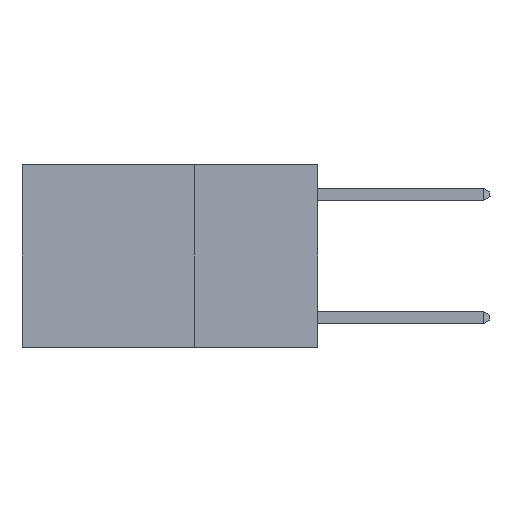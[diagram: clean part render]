
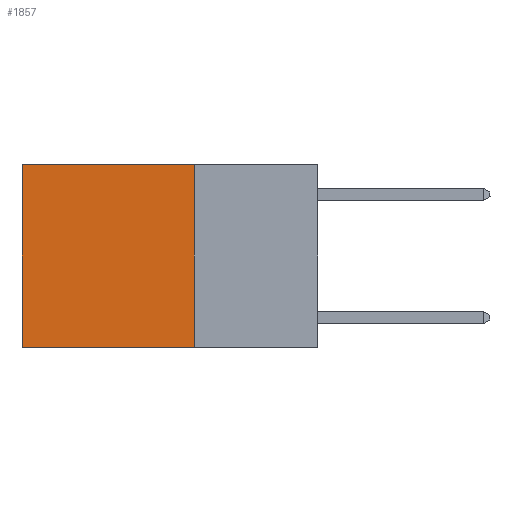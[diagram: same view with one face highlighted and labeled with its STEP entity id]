
A CAD part, left-side view. The second image highlights one B-rep face of the part: STEP entity #1857.
In plain terms, the highlighted planar face has unit normal (-1, 0, 0).
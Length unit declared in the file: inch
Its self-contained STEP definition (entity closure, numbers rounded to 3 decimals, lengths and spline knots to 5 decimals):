
#197 = CARTESIAN_POINT ( 'NONE',  ( 0.2625, 0.25, -0.37 ) ) ;
#1006 = LINE ( 'NONE', #4265, #3713 ) ;
#1363 = CARTESIAN_POINT ( 'NONE',  ( 0.2625, 0.6, 0. ) ) ;
#1785 = VERTEX_POINT ( 'NONE', #4185 ) ;
#1834 = EDGE_CURVE ( 'NONE', #1892, #7029, #1006, .T. ) ;
#1857 = ADVANCED_FACE ( 'NONE', ( #3415 ), #8069, .F. ) ;
#1885 = DIRECTION ( 'NONE',  ( 0., 1., 0. ) ) ;
#1892 = VERTEX_POINT ( 'NONE', #1363 ) ;
#1935 = VERTEX_POINT ( 'NONE', #9194 ) ;
#2248 = DIRECTION ( 'NONE',  ( 0., 0., -1. ) ) ;
#2295 = CARTESIAN_POINT ( 'NONE',  ( 0.2625, 0.25, 0. ) ) ;
#2737 = ORIENTED_EDGE ( 'NONE', *, *, #3218, .T. ) ;
#3174 = LINE ( 'NONE', #197, #4089 ) ;
#3218 = EDGE_CURVE ( 'NONE', #1935, #1892, #4878, .T. ) ;
#3338 = DIRECTION ( 'NONE',  ( 1., 0., 0. ) ) ;
#3415 = FACE_OUTER_BOUND ( 'NONE', #7387, .T. ) ;
#3713 = VECTOR ( 'NONE', #2248, 39.37008 ) ;
#3817 = DIRECTION ( 'NONE',  ( 0., 0., -1. ) ) ;
#3826 = EDGE_CURVE ( 'NONE', #1935, #1785, #7539, .T. ) ;
#4089 = VECTOR ( 'NONE', #6153, 39.37008 ) ;
#4185 = CARTESIAN_POINT ( 'NONE',  ( 0.2625, 0.25, -0.37 ) ) ;
#4265 = CARTESIAN_POINT ( 'NONE',  ( 0.2625, 0.6, 0. ) ) ;
#4835 = EDGE_CURVE ( 'NONE', #1785, #7029, #3174, .T. ) ;
#4878 = LINE ( 'NONE', #7699, #12189 ) ;
#4955 = AXIS2_PLACEMENT_3D ( 'NONE', #2295, #3338, #10030 ) ;
#6153 = DIRECTION ( 'NONE',  ( 0., 1., 0. ) ) ;
#7029 = VERTEX_POINT ( 'NONE', #11890 ) ;
#7387 = EDGE_LOOP ( 'NONE', ( #9165, #10460, #10352, #2737 ) ) ;
#7539 = LINE ( 'NONE', #8513, #12323 ) ;
#7699 = CARTESIAN_POINT ( 'NONE',  ( 0.2625, 0.25, 0. ) ) ;
#8069 = PLANE ( 'NONE',  #4955 ) ;
#8513 = CARTESIAN_POINT ( 'NONE',  ( 0.2625, 0.25, 0. ) ) ;
#9165 = ORIENTED_EDGE ( 'NONE', *, *, #1834, .T. ) ;
#9194 = CARTESIAN_POINT ( 'NONE',  ( 0.2625, 0.25, 0. ) ) ;
#10030 = DIRECTION ( 'NONE',  ( 0., 0., -1. ) ) ;
#10352 = ORIENTED_EDGE ( 'NONE', *, *, #3826, .F. ) ;
#10460 = ORIENTED_EDGE ( 'NONE', *, *, #4835, .F. ) ;
#11890 = CARTESIAN_POINT ( 'NONE',  ( 0.2625, 0.6, -0.37 ) ) ;
#12189 = VECTOR ( 'NONE', #1885, 39.37008 ) ;
#12323 = VECTOR ( 'NONE', #3817, 39.37008 ) ;
